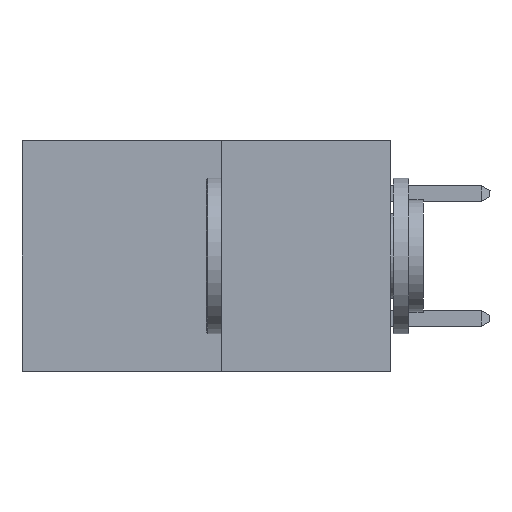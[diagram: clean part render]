
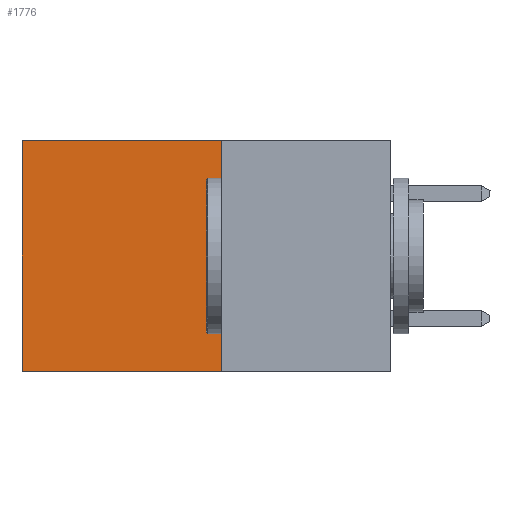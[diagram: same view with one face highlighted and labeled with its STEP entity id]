
A CAD part, left-side view. The second image highlights one B-rep face of the part: STEP entity #1776.
In plain terms, the highlighted planar face has unit normal (-1, 0, 0).
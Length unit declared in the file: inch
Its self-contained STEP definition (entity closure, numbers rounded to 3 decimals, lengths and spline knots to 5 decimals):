
#71 = DIRECTION ( 'NONE',  ( 0., 0., -1. ) ) ;
#159 = VERTEX_POINT ( 'NONE', #11363 ) ;
#226 = EDGE_CURVE ( 'NONE', #159, #2140, #6338, .T. ) ;
#884 = EDGE_LOOP ( 'NONE', ( #10188, #7955, #11569, #7802 ) ) ;
#976 = AXIS2_PLACEMENT_3D ( 'NONE', #4643, #5249, #4156 ) ;
#1355 = LINE ( 'NONE', #8210, #6201 ) ;
#1748 = CARTESIAN_POINT ( 'NONE',  ( 0.277, 0.27, -0.37 ) ) ;
#1776 = ADVANCED_FACE ( 'NONE', ( #6595 ), #4779, .F. ) ;
#2140 = VERTEX_POINT ( 'NONE', #3230 ) ;
#2517 = EDGE_CURVE ( 'NONE', #159, #7245, #11395, .T. ) ;
#3230 = CARTESIAN_POINT ( 'NONE',  ( 0.277, 0.59, 0. ) ) ;
#3730 = VECTOR ( 'NONE', #5911, 39.37008 ) ;
#3920 = CARTESIAN_POINT ( 'NONE',  ( 0.277, 0.27, -0.37 ) ) ;
#3930 = CARTESIAN_POINT ( 'NONE',  ( 0.277, 0.59, -0.37 ) ) ;
#4156 = DIRECTION ( 'NONE',  ( 0., 0., -1. ) ) ;
#4222 = LINE ( 'NONE', #1748, #6845 ) ;
#4643 = CARTESIAN_POINT ( 'NONE',  ( 0.277, 0.27, -0.37 ) ) ;
#4779 = PLANE ( 'NONE',  #976 ) ;
#5249 = DIRECTION ( 'NONE',  ( 1., 0., 0. ) ) ;
#5641 = CARTESIAN_POINT ( 'NONE',  ( 0.277, 0.27, -0.37 ) ) ;
#5648 = EDGE_CURVE ( 'NONE', #2140, #12633, #1355, .T. ) ;
#5911 = DIRECTION ( 'NONE',  ( 0., 0., -1. ) ) ;
#6201 = VECTOR ( 'NONE', #71, 39.37008 ) ;
#6338 = LINE ( 'NONE', #6933, #8583 ) ;
#6595 = FACE_OUTER_BOUND ( 'NONE', #884, .T. ) ;
#6845 = VECTOR ( 'NONE', #8776, 39.37008 ) ;
#6933 = CARTESIAN_POINT ( 'NONE',  ( 0.277, 0.27, 0. ) ) ;
#7194 = DIRECTION ( 'NONE',  ( 0., 1., 0. ) ) ;
#7245 = VERTEX_POINT ( 'NONE', #3920 ) ;
#7802 = ORIENTED_EDGE ( 'NONE', *, *, #226, .T. ) ;
#7955 = ORIENTED_EDGE ( 'NONE', *, *, #12579, .F. ) ;
#8210 = CARTESIAN_POINT ( 'NONE',  ( 0.277, 0.59, -0.37 ) ) ;
#8583 = VECTOR ( 'NONE', #7194, 39.37008 ) ;
#8776 = DIRECTION ( 'NONE',  ( 0., 1., 0. ) ) ;
#10188 = ORIENTED_EDGE ( 'NONE', *, *, #5648, .T. ) ;
#11363 = CARTESIAN_POINT ( 'NONE',  ( 0.277, 0.27, 0. ) ) ;
#11395 = LINE ( 'NONE', #5641, #3730 ) ;
#11569 = ORIENTED_EDGE ( 'NONE', *, *, #2517, .F. ) ;
#12579 = EDGE_CURVE ( 'NONE', #7245, #12633, #4222, .T. ) ;
#12633 = VERTEX_POINT ( 'NONE', #3930 ) ;
